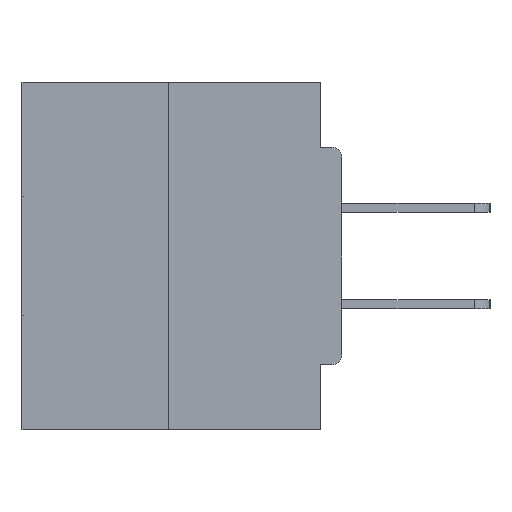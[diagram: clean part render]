
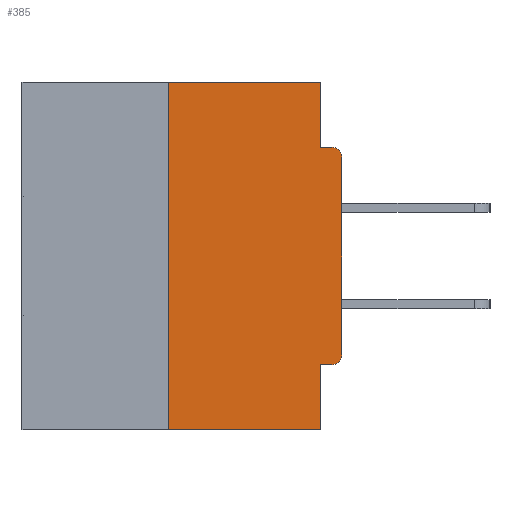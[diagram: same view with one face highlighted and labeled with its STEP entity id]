
A CAD part, left-side view. The second image highlights one B-rep face of the part: STEP entity #385.
In plain terms, the highlighted planar face has unit normal (-1, 0, 0).
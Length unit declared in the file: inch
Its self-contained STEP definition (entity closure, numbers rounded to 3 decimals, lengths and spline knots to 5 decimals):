
#247 = CARTESIAN_POINT ( 'NONE',  ( 0., 0.031, -0.5 ) ) ;
#370 = LINE ( 'NONE', #34891, #29616 ) ;
#385 = ADVANCED_FACE ( 'NONE', ( #37920 ), #29239, .F. ) ;
#1198 = CARTESIAN_POINT ( 'NONE',  ( 0., 0., -0.0935 ) ) ;
#2323 = CARTESIAN_POINT ( 'NONE',  ( 0., 0.031, -0.0935 ) ) ;
#2486 = DIRECTION ( 'NONE',  ( 0., 0., -1. ) ) ;
#2487 = EDGE_CURVE ( 'NONE', #10606, #32365, #11146, .T. ) ;
#2526 = EDGE_CURVE ( 'NONE', #5866, #25603, #6144, .T. ) ;
#2819 = CARTESIAN_POINT ( 'NONE',  ( 0., 0.46, 0. ) ) ;
#3235 = ORIENTED_EDGE ( 'NONE', *, *, #9547, .T. ) ;
#3481 = VECTOR ( 'NONE', #5948, 39.37008 ) ;
#4109 = CARTESIAN_POINT ( 'NONE',  ( 0., 0.46, 0. ) ) ;
#5664 = LINE ( 'NONE', #6048, #23161 ) ;
#5866 = VERTEX_POINT ( 'NONE', #26136 ) ;
#5871 = CARTESIAN_POINT ( 'NONE',  ( 0., 0.25, 0. ) ) ;
#5948 = DIRECTION ( 'NONE',  ( 0., 0., 1. ) ) ;
#6048 = CARTESIAN_POINT ( 'NONE',  ( 0., 0., -0.4065 ) ) ;
#6144 = CIRCLE ( 'NONE', #25873, 0.015 ) ;
#7034 = CARTESIAN_POINT ( 'NONE',  ( 0., 0.25, -0.5 ) ) ;
#7912 = CARTESIAN_POINT ( 'NONE',  ( 0., 0.46, -0.5 ) ) ;
#8210 = DIRECTION ( 'NONE',  ( 0., 0., -1. ) ) ;
#8460 = CARTESIAN_POINT ( 'NONE',  ( 0., 0.015, -0.1085 ) ) ;
#8900 = DIRECTION ( 'NONE',  ( 0., 0., -1. ) ) ;
#9072 = AXIS2_PLACEMENT_3D ( 'NONE', #2819, #22882, #34658 ) ;
#9186 = ORIENTED_EDGE ( 'NONE', *, *, #16283, .F. ) ;
#9547 = EDGE_CURVE ( 'NONE', #31996, #20949, #24425, .T. ) ;
#9738 = VERTEX_POINT ( 'NONE', #5871 ) ;
#10606 = VERTEX_POINT ( 'NONE', #35408 ) ;
#11146 = LINE ( 'NONE', #11706, #32016 ) ;
#11706 = CARTESIAN_POINT ( 'NONE',  ( 0., 0.031, -0.5 ) ) ;
#12377 = LINE ( 'NONE', #4109, #15554 ) ;
#13115 = DIRECTION ( 'NONE',  ( 0., -1., 0. ) ) ;
#13543 = VERTEX_POINT ( 'NONE', #7034 ) ;
#14756 = VECTOR ( 'NONE', #8900, 39.37008 ) ;
#15278 = EDGE_CURVE ( 'NONE', #34443, #25603, #27594, .T. ) ;
#15554 = VECTOR ( 'NONE', #24336, 39.37008 ) ;
#16283 = EDGE_CURVE ( 'NONE', #36557, #34443, #35307, .T. ) ;
#17268 = ORIENTED_EDGE ( 'NONE', *, *, #32150, .F. ) ;
#17347 = DIRECTION ( 'NONE',  ( 0., 0., 1. ) ) ;
#17432 = EDGE_CURVE ( 'NONE', #20949, #5866, #370, .T. ) ;
#17701 = CARTESIAN_POINT ( 'NONE',  ( 0., 0.25, 0. ) ) ;
#17819 = CARTESIAN_POINT ( 'NONE',  ( 0., 0., -0.3915 ) ) ;
#19181 = CARTESIAN_POINT ( 'NONE',  ( 0., 0.015, -0.4065 ) ) ;
#20478 = ORIENTED_EDGE ( 'NONE', *, *, #24872, .F. ) ;
#20949 = VERTEX_POINT ( 'NONE', #17819 ) ;
#21201 = CARTESIAN_POINT ( 'NONE',  ( 0., 0.031, 0. ) ) ;
#22721 = DIRECTION ( 'NONE',  ( -1., 0., 0. ) ) ;
#22845 = DIRECTION ( 'NONE',  ( -1., 0., 0. ) ) ;
#22882 = DIRECTION ( 'NONE',  ( 1., 0., 0. ) ) ;
#23161 = VECTOR ( 'NONE', #32251, 39.37008 ) ;
#23285 = DIRECTION ( 'NONE',  ( 0., 0., -1. ) ) ;
#23308 = VECTOR ( 'NONE', #28164, 39.37008 ) ;
#24336 = DIRECTION ( 'NONE',  ( 0., -1., 0. ) ) ;
#24425 = CIRCLE ( 'NONE', #25039, 0.015 ) ;
#24684 = EDGE_CURVE ( 'NONE', #13543, #32365, #33752, .T. ) ;
#24827 = ORIENTED_EDGE ( 'NONE', *, *, #15278, .F. ) ;
#24872 = EDGE_CURVE ( 'NONE', #13543, #9738, #32346, .T. ) ;
#25039 = AXIS2_PLACEMENT_3D ( 'NONE', #30399, #22845, #8210 ) ;
#25603 = VERTEX_POINT ( 'NONE', #27752 ) ;
#25873 = AXIS2_PLACEMENT_3D ( 'NONE', #8460, #22721, #2486 ) ;
#25988 = ORIENTED_EDGE ( 'NONE', *, *, #28375, .F. ) ;
#26136 = CARTESIAN_POINT ( 'NONE',  ( 0., 0., -0.1085 ) ) ;
#26449 = CARTESIAN_POINT ( 'NONE',  ( 0., 0.031, 0. ) ) ;
#27594 = LINE ( 'NONE', #1198, #23308 ) ;
#27752 = CARTESIAN_POINT ( 'NONE',  ( 0., 0.015, -0.0935 ) ) ;
#28164 = DIRECTION ( 'NONE',  ( 0., -1., 0. ) ) ;
#28354 = ORIENTED_EDGE ( 'NONE', *, *, #17432, .T. ) ;
#28375 = EDGE_CURVE ( 'NONE', #9738, #36557, #12377, .T. ) ;
#29239 = PLANE ( 'NONE',  #9072 ) ;
#29616 = VECTOR ( 'NONE', #17347, 39.37008 ) ;
#30399 = CARTESIAN_POINT ( 'NONE',  ( 0., 0.015, -0.3915 ) ) ;
#31173 = ORIENTED_EDGE ( 'NONE', *, *, #2526, .T. ) ;
#31780 = ORIENTED_EDGE ( 'NONE', *, *, #2487, .F. ) ;
#31996 = VERTEX_POINT ( 'NONE', #19181 ) ;
#32016 = VECTOR ( 'NONE', #23285, 39.37008 ) ;
#32150 = EDGE_CURVE ( 'NONE', #31996, #10606, #5664, .T. ) ;
#32251 = DIRECTION ( 'NONE',  ( 0., 1., 0. ) ) ;
#32346 = LINE ( 'NONE', #17701, #3481 ) ;
#32365 = VERTEX_POINT ( 'NONE', #247 ) ;
#33285 = EDGE_LOOP ( 'NONE', ( #25988, #20478, #36008, #31780, #17268, #3235, #28354, #31173, #24827, #9186 ) ) ;
#33752 = LINE ( 'NONE', #7912, #36678 ) ;
#34443 = VERTEX_POINT ( 'NONE', #2323 ) ;
#34658 = DIRECTION ( 'NONE',  ( 0., 0., -1. ) ) ;
#34891 = CARTESIAN_POINT ( 'NONE',  ( 0., 0., 0. ) ) ;
#35307 = LINE ( 'NONE', #26449, #14756 ) ;
#35408 = CARTESIAN_POINT ( 'NONE',  ( 0., 0.031, -0.4065 ) ) ;
#36008 = ORIENTED_EDGE ( 'NONE', *, *, #24684, .T. ) ;
#36557 = VERTEX_POINT ( 'NONE', #21201 ) ;
#36678 = VECTOR ( 'NONE', #13115, 39.37008 ) ;
#37920 = FACE_OUTER_BOUND ( 'NONE', #33285, .T. ) ;
